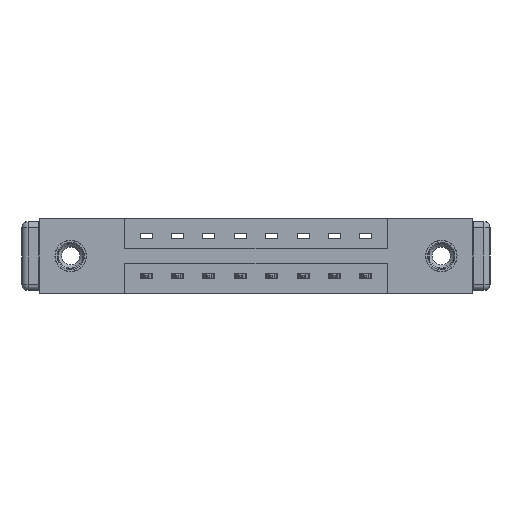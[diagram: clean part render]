
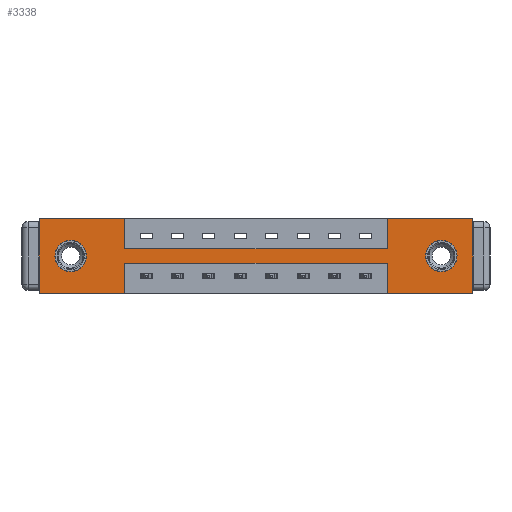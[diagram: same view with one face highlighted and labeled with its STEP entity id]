
A CAD part, front view. The second image highlights one B-rep face of the part: STEP entity #3338.
In plain terms, the highlighted planar face has unit normal (0, -1, 0).
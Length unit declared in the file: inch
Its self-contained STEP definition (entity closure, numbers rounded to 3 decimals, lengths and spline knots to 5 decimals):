
#57 = CARTESIAN_POINT ( 'NONE',  ( 0.425, 0., -0.22 ) ) ;
#264 = AXIS2_PLACEMENT_3D ( 'NONE', #12793, #10726, #6758 ) ;
#309 = EDGE_CURVE ( 'NONE', #9870, #1253, #9364, .T. ) ;
#352 = DIRECTION ( 'NONE',  ( -1., 0., 0. ) ) ;
#419 = AXIS2_PLACEMENT_3D ( 'NONE', #8426, #2322, #4480 ) ;
#436 = AXIS2_PLACEMENT_3D ( 'NONE', #7673, #1694, #2733 ) ;
#627 = VERTEX_POINT ( 'NONE', #7799 ) ;
#762 = CARTESIAN_POINT ( 'NONE',  ( 0., 0., -0.37 ) ) ;
#813 = VERTEX_POINT ( 'NONE', #8147 ) ;
#1148 = CARTESIAN_POINT ( 'NONE',  ( 1.729, 0., 0. ) ) ;
#1170 = CARTESIAN_POINT ( 'NONE',  ( 0., 0., 0. ) ) ;
#1172 = FACE_BOUND ( 'NONE', #4013, .T. ) ;
#1253 = VERTEX_POINT ( 'NONE', #8150 ) ;
#1618 = EDGE_CURVE ( 'NONE', #813, #3806, #3770, .T. ) ;
#1681 = ORIENTED_EDGE ( 'NONE', *, *, #6152, .F. ) ;
#1694 = DIRECTION ( 'NONE',  ( 0., -1., 0. ) ) ;
#1774 = FACE_BOUND ( 'NONE', #4208, .T. ) ;
#2032 = EDGE_CURVE ( 'NONE', #2034, #10665, #6457, .T. ) ;
#2034 = VERTEX_POINT ( 'NONE', #4165 ) ;
#2088 = EDGE_CURVE ( 'NONE', #7195, #2034, #11550, .T. ) ;
#2098 = VERTEX_POINT ( 'NONE', #3363 ) ;
#2287 = ORIENTED_EDGE ( 'NONE', *, *, #8117, .T. ) ;
#2322 = DIRECTION ( 'NONE',  ( 0., 1., 0. ) ) ;
#2733 = DIRECTION ( 'NONE',  ( 0., 0., -1. ) ) ;
#2810 = ORIENTED_EDGE ( 'NONE', *, *, #2977, .T. ) ;
#2831 = AXIS2_PLACEMENT_3D ( 'NONE', #8803, #5686, #9821 ) ;
#2913 = CARTESIAN_POINT ( 'NONE',  ( 1.999, 0., -0.263 ) ) ;
#2977 = EDGE_CURVE ( 'NONE', #8309, #2098, #10582, .T. ) ;
#3279 = CARTESIAN_POINT ( 'NONE',  ( 2.154, 0., 0. ) ) ;
#3285 = EDGE_LOOP ( 'NONE', ( #3523, #11851, #5493, #12526, #10152, #7679, #9525, #12093, #9674, #11821, #6119, #1681 ) ) ;
#3338 = ADVANCED_FACE ( 'NONE', ( #1172, #1774, #7046 ), #12856, .T. ) ;
#3363 = CARTESIAN_POINT ( 'NONE',  ( 1.999, 0., -0.107 ) ) ;
#3368 = CARTESIAN_POINT ( 'NONE',  ( 0.425, 0., -0.15 ) ) ;
#3398 = CARTESIAN_POINT ( 'NONE',  ( 0.425, 0., -0.37 ) ) ;
#3416 = EDGE_CURVE ( 'NONE', #12395, #627, #8808, .T. ) ;
#3523 = ORIENTED_EDGE ( 'NONE', *, *, #7975, .F. ) ;
#3569 = LINE ( 'NONE', #3398, #11028 ) ;
#3674 = VECTOR ( 'NONE', #352, 39.37008 ) ;
#3770 = CIRCLE ( 'NONE', #419, 0.078 ) ;
#3798 = CARTESIAN_POINT ( 'NONE',  ( 0., 0., 0. ) ) ;
#3806 = VERTEX_POINT ( 'NONE', #12052 ) ;
#4013 = EDGE_LOOP ( 'NONE', ( #5410, #2810 ) ) ;
#4018 = DIRECTION ( 'NONE',  ( -1., 0., 0. ) ) ;
#4165 = CARTESIAN_POINT ( 'NONE',  ( 0.425, 0., 0. ) ) ;
#4207 = LINE ( 'NONE', #4382, #11520 ) ;
#4208 = EDGE_LOOP ( 'NONE', ( #2287, #11914 ) ) ;
#4382 = CARTESIAN_POINT ( 'NONE',  ( 0.425, 0., -0.15 ) ) ;
#4441 = VERTEX_POINT ( 'NONE', #12981 ) ;
#4480 = DIRECTION ( 'NONE',  ( 0., 0., 1. ) ) ;
#4569 = VECTOR ( 'NONE', #9586, 39.37008 ) ;
#4974 = CARTESIAN_POINT ( 'NONE',  ( 1.729, 0., -0.37 ) ) ;
#5093 = LINE ( 'NONE', #762, #12270 ) ;
#5379 = DIRECTION ( 'NONE',  ( 1., 0., 0. ) ) ;
#5410 = ORIENTED_EDGE ( 'NONE', *, *, #10875, .T. ) ;
#5493 = ORIENTED_EDGE ( 'NONE', *, *, #8352, .F. ) ;
#5500 = CARTESIAN_POINT ( 'NONE',  ( 0., 0., -0.37 ) ) ;
#5550 = VERTEX_POINT ( 'NONE', #4974 ) ;
#5686 = DIRECTION ( 'NONE',  ( 0., 1., 0. ) ) ;
#5867 = LINE ( 'NONE', #5500, #3674 ) ;
#6119 = ORIENTED_EDGE ( 'NONE', *, *, #12468, .F. ) ;
#6152 = EDGE_CURVE ( 'NONE', #4441, #7721, #5093, .T. ) ;
#6173 = CARTESIAN_POINT ( 'NONE',  ( 1.729, 0., -0.37 ) ) ;
#6457 = LINE ( 'NONE', #12734, #12660 ) ;
#6550 = VECTOR ( 'NONE', #9241, 39.37008 ) ;
#6652 = VECTOR ( 'NONE', #13117, 39.37008 ) ;
#6758 = DIRECTION ( 'NONE',  ( 0., 0., -1. ) ) ;
#6800 = VERTEX_POINT ( 'NONE', #1148 ) ;
#6947 = EDGE_CURVE ( 'NONE', #6800, #12395, #10984, .T. ) ;
#7046 = FACE_OUTER_BOUND ( 'NONE', #3285, .T. ) ;
#7195 = VERTEX_POINT ( 'NONE', #3798 ) ;
#7214 = CARTESIAN_POINT ( 'NONE',  ( 1.729, 0., 0. ) ) ;
#7518 = CARTESIAN_POINT ( 'NONE',  ( 0., 0., -0.37 ) ) ;
#7647 = DIRECTION ( 'NONE',  ( 0., 0., -1. ) ) ;
#7673 = CARTESIAN_POINT ( 'NONE',  ( 0., 0., -0.37 ) ) ;
#7679 = ORIENTED_EDGE ( 'NONE', *, *, #6947, .F. ) ;
#7721 = VERTEX_POINT ( 'NONE', #7518 ) ;
#7799 = CARTESIAN_POINT ( 'NONE',  ( 2.154, 0., -0.37 ) ) ;
#7821 = DIRECTION ( 'NONE',  ( 0., 1., 0. ) ) ;
#7975 = EDGE_CURVE ( 'NONE', #1253, #4441, #3569, .T. ) ;
#8117 = EDGE_CURVE ( 'NONE', #3806, #813, #12441, .T. ) ;
#8147 = CARTESIAN_POINT ( 'NONE',  ( 0.155, 0., -0.263 ) ) ;
#8150 = CARTESIAN_POINT ( 'NONE',  ( 0.425, 0., -0.22 ) ) ;
#8309 = VERTEX_POINT ( 'NONE', #2913 ) ;
#8352 = EDGE_CURVE ( 'NONE', #5550, #9870, #13033, .T. ) ;
#8412 = CARTESIAN_POINT ( 'NONE',  ( 1.729, 0., -0.22 ) ) ;
#8426 = CARTESIAN_POINT ( 'NONE',  ( 0.155, 0., -0.185 ) ) ;
#8803 = CARTESIAN_POINT ( 'NONE',  ( 0.155, 0., -0.185 ) ) ;
#8808 = LINE ( 'NONE', #9991, #12011 ) ;
#8894 = VECTOR ( 'NONE', #10806, 39.37008 ) ;
#9028 = CARTESIAN_POINT ( 'NONE',  ( 0., 0., 0. ) ) ;
#9059 = EDGE_CURVE ( 'NONE', #12720, #6800, #11142, .T. ) ;
#9241 = DIRECTION ( 'NONE',  ( 0., 0., 1. ) ) ;
#9278 = DIRECTION ( 'NONE',  ( 0., 0., 1. ) ) ;
#9364 = LINE ( 'NONE', #57, #6652 ) ;
#9525 = ORIENTED_EDGE ( 'NONE', *, *, #9059, .F. ) ;
#9586 = DIRECTION ( 'NONE',  ( 1., 0., 0. ) ) ;
#9674 = ORIENTED_EDGE ( 'NONE', *, *, #2032, .F. ) ;
#9765 = CARTESIAN_POINT ( 'NONE',  ( 1.999, 0., -0.185 ) ) ;
#9821 = DIRECTION ( 'NONE',  ( 0., 0., 1. ) ) ;
#9870 = VERTEX_POINT ( 'NONE', #8412 ) ;
#9991 = CARTESIAN_POINT ( 'NONE',  ( 2.154, 0., 0. ) ) ;
#10152 = ORIENTED_EDGE ( 'NONE', *, *, #3416, .F. ) ;
#10207 = DIRECTION ( 'NONE',  ( 0., 0., -1. ) ) ;
#10445 = EDGE_CURVE ( 'NONE', #627, #5550, #5867, .T. ) ;
#10582 = CIRCLE ( 'NONE', #264, 0.078 ) ;
#10665 = VERTEX_POINT ( 'NONE', #3368 ) ;
#10690 = LINE ( 'NONE', #9028, #11327 ) ;
#10726 = DIRECTION ( 'NONE',  ( 0., 1., 0. ) ) ;
#10806 = DIRECTION ( 'NONE',  ( 1., 0., 0. ) ) ;
#10875 = EDGE_CURVE ( 'NONE', #2098, #8309, #12689, .T. ) ;
#10984 = LINE ( 'NONE', #11466, #8894 ) ;
#11028 = VECTOR ( 'NONE', #11301, 39.37008 ) ;
#11121 = DIRECTION ( 'NONE',  ( 0., 0., 1. ) ) ;
#11142 = LINE ( 'NONE', #7214, #12865 ) ;
#11301 = DIRECTION ( 'NONE',  ( 0., 0., -1. ) ) ;
#11327 = VECTOR ( 'NONE', #11121, 39.37008 ) ;
#11466 = CARTESIAN_POINT ( 'NONE',  ( 0., 0., 0. ) ) ;
#11520 = VECTOR ( 'NONE', #5379, 39.37008 ) ;
#11535 = EDGE_CURVE ( 'NONE', #10665, #12720, #4207, .T. ) ;
#11550 = LINE ( 'NONE', #1170, #4569 ) ;
#11663 = AXIS2_PLACEMENT_3D ( 'NONE', #9765, #7821, #7647 ) ;
#11821 = ORIENTED_EDGE ( 'NONE', *, *, #2088, .F. ) ;
#11851 = ORIENTED_EDGE ( 'NONE', *, *, #309, .F. ) ;
#11914 = ORIENTED_EDGE ( 'NONE', *, *, #1618, .T. ) ;
#12011 = VECTOR ( 'NONE', #12048, 39.37008 ) ;
#12048 = DIRECTION ( 'NONE',  ( 0., 0., -1. ) ) ;
#12052 = CARTESIAN_POINT ( 'NONE',  ( 0.155, 0., -0.107 ) ) ;
#12093 = ORIENTED_EDGE ( 'NONE', *, *, #11535, .F. ) ;
#12270 = VECTOR ( 'NONE', #4018, 39.37008 ) ;
#12395 = VERTEX_POINT ( 'NONE', #3279 ) ;
#12441 = CIRCLE ( 'NONE', #2831, 0.078 ) ;
#12468 = EDGE_CURVE ( 'NONE', #7721, #7195, #10690, .T. ) ;
#12489 = CARTESIAN_POINT ( 'NONE',  ( 1.729, 0., -0.15 ) ) ;
#12526 = ORIENTED_EDGE ( 'NONE', *, *, #10445, .F. ) ;
#12660 = VECTOR ( 'NONE', #10207, 39.37008 ) ;
#12689 = CIRCLE ( 'NONE', #11663, 0.078 ) ;
#12720 = VERTEX_POINT ( 'NONE', #12489 ) ;
#12734 = CARTESIAN_POINT ( 'NONE',  ( 0.425, 0., 0. ) ) ;
#12793 = CARTESIAN_POINT ( 'NONE',  ( 1.999, 0., -0.185 ) ) ;
#12856 = PLANE ( 'NONE',  #436 ) ;
#12865 = VECTOR ( 'NONE', #9278, 39.37008 ) ;
#12981 = CARTESIAN_POINT ( 'NONE',  ( 0.425, 0., -0.37 ) ) ;
#13033 = LINE ( 'NONE', #6173, #6550 ) ;
#13117 = DIRECTION ( 'NONE',  ( -1., 0., 0. ) ) ;
